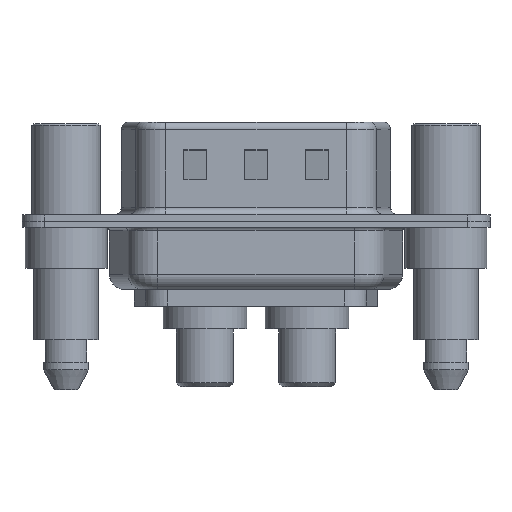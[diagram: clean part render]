
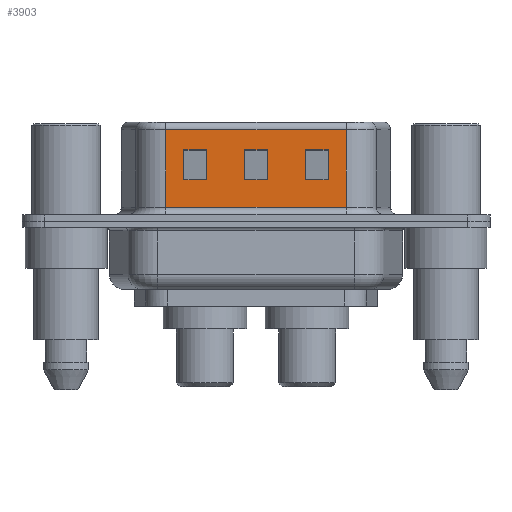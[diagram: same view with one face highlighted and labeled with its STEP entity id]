
A CAD part, front view. The second image highlights one B-rep face of the part: STEP entity #3903.
In plain terms, the highlighted planar face has unit normal (0, -1, 0).
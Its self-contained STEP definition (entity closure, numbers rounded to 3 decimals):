
#67 = VECTOR ( 'NONE', #11130, 1000. ) ;
#211 = DIRECTION ( 'NONE',  ( 0., 0., -1. ) ) ;
#273 = CARTESIAN_POINT ( 'NONE',  ( 15.75, -4.58, 2.705 ) ) ;
#336 = ORIENTED_EDGE ( 'NONE', *, *, #11042, .T. ) ;
#384 = DIRECTION ( 'NONE',  ( 0., 0., -1. ) ) ;
#429 = ORIENTED_EDGE ( 'NONE', *, *, #10618, .T. ) ;
#893 = CARTESIAN_POINT ( 'NONE',  ( 13.25, -4.58, 4.705 ) ) ;
#1014 = LINE ( 'NONE', #10457, #6863 ) ;
#1022 = VECTOR ( 'NONE', #384, 1000. ) ;
#1211 = VERTEX_POINT ( 'NONE', #6227 ) ;
#1389 = CARTESIAN_POINT ( 'NONE',  ( 18.45, -4.58, 6.52 ) ) ;
#1568 = VERTEX_POINT ( 'NONE', #893 ) ;
#1750 = LINE ( 'NONE', #10745, #13354 ) ;
#1899 = CARTESIAN_POINT ( 'NONE',  ( 18.45, -4.58, 0.9 ) ) ;
#1941 = CARTESIAN_POINT ( 'NONE',  ( 7.75, -4.58, 2.705 ) ) ;
#2044 = LINE ( 'NONE', #5673, #7857 ) ;
#2076 = CARTESIAN_POINT ( 'NONE',  ( 9.25, -4.58, 4.705 ) ) ;
#2539 = VERTEX_POINT ( 'NONE', #273 ) ;
#2549 = VERTEX_POINT ( 'NONE', #7951 ) ;
#2646 = CARTESIAN_POINT ( 'NONE',  ( 13.25, -4.58, 2.705 ) ) ;
#2712 = VERTEX_POINT ( 'NONE', #3787 ) ;
#2716 = VERTEX_POINT ( 'NONE', #9208 ) ;
#2857 = LINE ( 'NONE', #5372, #8692 ) ;
#2858 = EDGE_CURVE ( 'NONE', #2549, #2712, #13121, .T. ) ;
#2893 = EDGE_LOOP ( 'NONE', ( #6845, #12617, #429, #7473 ) ) ;
#2968 = CARTESIAN_POINT ( 'NONE',  ( 11.75, -4.58, 6.52 ) ) ;
#3009 = EDGE_CURVE ( 'NONE', #2549, #6131, #2044, .T. ) ;
#3038 = DIRECTION ( 'NONE',  ( -1., 0., 0. ) ) ;
#3274 = DIRECTION ( 'NONE',  ( 0., 0., 1. ) ) ;
#3316 = VECTOR ( 'NONE', #13109, 1000. ) ;
#3375 = DIRECTION ( 'NONE',  ( -1., 0., 0. ) ) ;
#3470 = ORIENTED_EDGE ( 'NONE', *, *, #12497, .T. ) ;
#3604 = ORIENTED_EDGE ( 'NONE', *, *, #10705, .T. ) ;
#3652 = CARTESIAN_POINT ( 'NONE',  ( 7.75, -4.58, 4.705 ) ) ;
#3787 = CARTESIAN_POINT ( 'NONE',  ( 18.45, -4.58, 0.9 ) ) ;
#3903 = ADVANCED_FACE ( 'NONE', ( #4167, #13004, #7553, #7196 ), #12292, .F. ) ;
#4147 = VECTOR ( 'NONE', #3274, 1000. ) ;
#4167 = FACE_BOUND ( 'NONE', #8303, .T. ) ;
#4360 = LINE ( 'NONE', #8817, #7045 ) ;
#4370 = CARTESIAN_POINT ( 'NONE',  ( 14.45, -4.58, 4.705 ) ) ;
#4640 = VECTOR ( 'NONE', #211, 1000. ) ;
#4958 = CARTESIAN_POINT ( 'NONE',  ( 18.45, -4.58, 6.52 ) ) ;
#5114 = VERTEX_POINT ( 'NONE', #2646 ) ;
#5149 = ORIENTED_EDGE ( 'NONE', *, *, #3009, .T. ) ;
#5262 = VECTOR ( 'NONE', #6067, 1000. ) ;
#5372 = CARTESIAN_POINT ( 'NONE',  ( 9.25, -4.58, 6.52 ) ) ;
#5415 = ORIENTED_EDGE ( 'NONE', *, *, #11319, .T. ) ;
#5673 = CARTESIAN_POINT ( 'NONE',  ( 18.45, -4.58, 6.02 ) ) ;
#5700 = DIRECTION ( 'NONE',  ( 0., 0., 1. ) ) ;
#6067 = DIRECTION ( 'NONE',  ( 1., 0., 0. ) ) ;
#6131 = VERTEX_POINT ( 'NONE', #12619 ) ;
#6156 = DIRECTION ( 'NONE',  ( 1., 0., 0. ) ) ;
#6227 = CARTESIAN_POINT ( 'NONE',  ( 17.25, -4.58, 4.705 ) ) ;
#6343 = LINE ( 'NONE', #8979, #67 ) ;
#6488 = DIRECTION ( 'NONE',  ( -1., 0., 0. ) ) ;
#6747 = CARTESIAN_POINT ( 'NONE',  ( 7.75, -4.58, 6.52 ) ) ;
#6797 = EDGE_LOOP ( 'NONE', ( #11141, #5149, #8040, #3604 ) ) ;
#6845 = ORIENTED_EDGE ( 'NONE', *, *, #10385, .T. ) ;
#6863 = VECTOR ( 'NONE', #8155, 1000. ) ;
#7045 = VECTOR ( 'NONE', #3038, 1000. ) ;
#7152 = DIRECTION ( 'NONE',  ( 0., 1., 0. ) ) ;
#7196 = FACE_OUTER_BOUND ( 'NONE', #6797, .T. ) ;
#7225 = LINE ( 'NONE', #13843, #1022 ) ;
#7420 = VECTOR ( 'NONE', #10151, 1000. ) ;
#7473 = ORIENTED_EDGE ( 'NONE', *, *, #10635, .T. ) ;
#7498 = VERTEX_POINT ( 'NONE', #12381 ) ;
#7536 = VERTEX_POINT ( 'NONE', #3652 ) ;
#7553 = FACE_BOUND ( 'NONE', #2893, .T. ) ;
#7857 = VECTOR ( 'NONE', #11930, 1000. ) ;
#7951 = CARTESIAN_POINT ( 'NONE',  ( 18.45, -4.58, 6.02 ) ) ;
#8040 = ORIENTED_EDGE ( 'NONE', *, *, #9937, .T. ) ;
#8155 = DIRECTION ( 'NONE',  ( 0., 0., -1. ) ) ;
#8303 = EDGE_LOOP ( 'NONE', ( #9677, #11946, #3470, #5415 ) ) ;
#8329 = VECTOR ( 'NONE', #3375, 1000. ) ;
#8336 = ORIENTED_EDGE ( 'NONE', *, *, #10725, .T. ) ;
#8397 = VERTEX_POINT ( 'NONE', #13177 ) ;
#8551 = LINE ( 'NONE', #11188, #7420 ) ;
#8692 = VECTOR ( 'NONE', #14176, 1000. ) ;
#8734 = LINE ( 'NONE', #11609, #5262 ) ;
#8817 = CARTESIAN_POINT ( 'NONE',  ( 18.45, -4.58, 2.705 ) ) ;
#8899 = VERTEX_POINT ( 'NONE', #10858 ) ;
#8979 = CARTESIAN_POINT ( 'NONE',  ( 15.75, -4.58, 6.52 ) ) ;
#9100 = VECTOR ( 'NONE', #12197, 1000. ) ;
#9141 = CARTESIAN_POINT ( 'NONE',  ( 9.25, -4.58, 2.705 ) ) ;
#9144 = CARTESIAN_POINT ( 'NONE',  ( 22.45, -4.58, 2.705 ) ) ;
#9208 = CARTESIAN_POINT ( 'NONE',  ( 17.25, -4.58, 2.705 ) ) ;
#9398 = VERTEX_POINT ( 'NONE', #1941 ) ;
#9424 = VERTEX_POINT ( 'NONE', #9141 ) ;
#9461 = LINE ( 'NONE', #4370, #9100 ) ;
#9609 = ORIENTED_EDGE ( 'NONE', *, *, #10261, .T. ) ;
#9677 = ORIENTED_EDGE ( 'NONE', *, *, #11882, .T. ) ;
#9837 = VECTOR ( 'NONE', #9996, 1000. ) ;
#9937 = EDGE_CURVE ( 'NONE', #6131, #8397, #8551, .T. ) ;
#9996 = DIRECTION ( 'NONE',  ( 0., 0., 1. ) ) ;
#10151 = DIRECTION ( 'NONE',  ( 0., 0., -1. ) ) ;
#10261 = EDGE_CURVE ( 'NONE', #8899, #1211, #8734, .T. ) ;
#10356 = AXIS2_PLACEMENT_3D ( 'NONE', #1389, #7152, #5700 ) ;
#10385 = EDGE_CURVE ( 'NONE', #7498, #1568, #1750, .T. ) ;
#10457 = CARTESIAN_POINT ( 'NONE',  ( 17.25, -4.58, 6.52 ) ) ;
#10462 = EDGE_CURVE ( 'NONE', #1568, #5114, #7225, .T. ) ;
#10618 = EDGE_CURVE ( 'NONE', #5114, #12067, #4360, .T. ) ;
#10635 = EDGE_CURVE ( 'NONE', #12067, #7498, #12568, .T. ) ;
#10705 = EDGE_CURVE ( 'NONE', #8397, #2712, #11925, .T. ) ;
#10725 = EDGE_CURVE ( 'NONE', #2539, #8899, #6343, .T. ) ;
#10745 = CARTESIAN_POINT ( 'NONE',  ( 18.45, -4.58, 4.705 ) ) ;
#10858 = CARTESIAN_POINT ( 'NONE',  ( 15.75, -4.58, 4.705 ) ) ;
#10885 = EDGE_CURVE ( 'NONE', #2716, #2539, #13680, .T. ) ;
#10929 = LINE ( 'NONE', #13055, #13626 ) ;
#11042 = EDGE_CURVE ( 'NONE', #1211, #2716, #1014, .T. ) ;
#11130 = DIRECTION ( 'NONE',  ( 0., 0., 1. ) ) ;
#11141 = ORIENTED_EDGE ( 'NONE', *, *, #2858, .F. ) ;
#11188 = CARTESIAN_POINT ( 'NONE',  ( 6.55, -4.58, 6.52 ) ) ;
#11319 = EDGE_CURVE ( 'NONE', #7536, #13850, #9461, .T. ) ;
#11609 = CARTESIAN_POINT ( 'NONE',  ( 22.45, -4.58, 4.705 ) ) ;
#11882 = EDGE_CURVE ( 'NONE', #13850, #9424, #2857, .T. ) ;
#11925 = LINE ( 'NONE', #1899, #3316 ) ;
#11930 = DIRECTION ( 'NONE',  ( -1., 0., 0. ) ) ;
#11946 = ORIENTED_EDGE ( 'NONE', *, *, #12960, .T. ) ;
#12067 = VERTEX_POINT ( 'NONE', #13438 ) ;
#12197 = DIRECTION ( 'NONE',  ( 1., 0., 0. ) ) ;
#12292 = PLANE ( 'NONE',  #10356 ) ;
#12381 = CARTESIAN_POINT ( 'NONE',  ( 11.75, -4.58, 4.705 ) ) ;
#12497 = EDGE_CURVE ( 'NONE', #9398, #7536, #13990, .T. ) ;
#12568 = LINE ( 'NONE', #2968, #9837 ) ;
#12617 = ORIENTED_EDGE ( 'NONE', *, *, #10462, .T. ) ;
#12619 = CARTESIAN_POINT ( 'NONE',  ( 6.55, -4.58, 6.02 ) ) ;
#12960 = EDGE_CURVE ( 'NONE', #9424, #9398, #10929, .T. ) ;
#12982 = ORIENTED_EDGE ( 'NONE', *, *, #10885, .T. ) ;
#13004 = FACE_BOUND ( 'NONE', #13682, .T. ) ;
#13055 = CARTESIAN_POINT ( 'NONE',  ( 14.45, -4.58, 2.705 ) ) ;
#13109 = DIRECTION ( 'NONE',  ( 1., 0., 0. ) ) ;
#13121 = LINE ( 'NONE', #4958, #4640 ) ;
#13177 = CARTESIAN_POINT ( 'NONE',  ( 6.55, -4.58, 0.9 ) ) ;
#13354 = VECTOR ( 'NONE', #6156, 1000. ) ;
#13438 = CARTESIAN_POINT ( 'NONE',  ( 11.75, -4.58, 2.705 ) ) ;
#13626 = VECTOR ( 'NONE', #6488, 1000. ) ;
#13680 = LINE ( 'NONE', #9144, #8329 ) ;
#13682 = EDGE_LOOP ( 'NONE', ( #336, #12982, #8336, #9609 ) ) ;
#13843 = CARTESIAN_POINT ( 'NONE',  ( 13.25, -4.58, 6.52 ) ) ;
#13850 = VERTEX_POINT ( 'NONE', #2076 ) ;
#13990 = LINE ( 'NONE', #6747, #4147 ) ;
#14176 = DIRECTION ( 'NONE',  ( 0., 0., -1. ) ) ;
